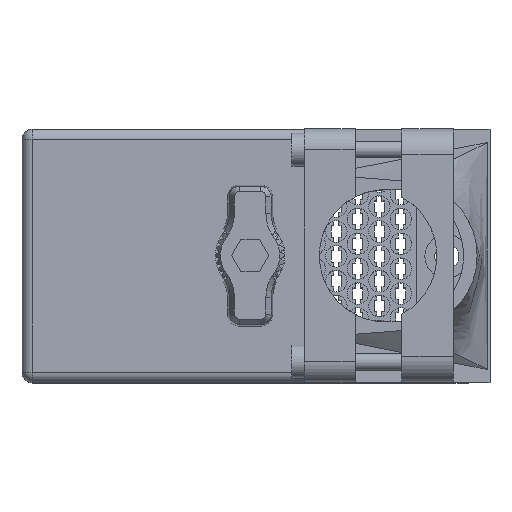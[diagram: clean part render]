
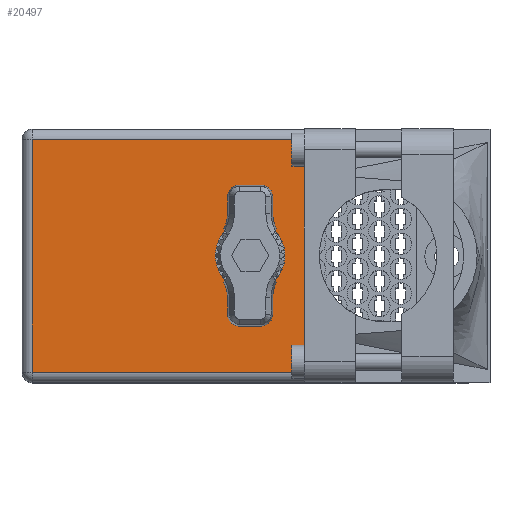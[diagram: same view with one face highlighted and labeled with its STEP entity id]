
A CAD part, top view. The second image highlights one B-rep face of the part: STEP entity #20497.
In plain terms, the highlighted face is planar.
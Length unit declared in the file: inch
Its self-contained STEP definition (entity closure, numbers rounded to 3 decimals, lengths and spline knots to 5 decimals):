
#471 = DIRECTION ( 'NONE',  ( 0., 1., 0. ) ) ;
#7063 = EDGE_CURVE ( 'NONE', #86197, #52435, #55895, .T. ) ;
#8745 = CIRCLE ( 'NONE', #77725, 0.1015 ) ;
#8870 = EDGE_CURVE ( 'NONE', #62942, #71681, #64493, .T. ) ;
#11421 = ORIENTED_EDGE ( 'NONE', *, *, #68523, .T. ) ;
#13861 = CARTESIAN_POINT ( 'NONE',  ( 1.705, 2.03, -1.468 ) ) ;
#15025 = CARTESIAN_POINT ( 'NONE',  ( 1.3775, 2.03, -0.8665 ) ) ;
#18262 = CARTESIAN_POINT ( 'NONE',  ( 0., 2.03, -1.53 ) ) ;
#19303 = DIRECTION ( 'NONE',  ( 0., 0., 1. ) ) ;
#19883 = CARTESIAN_POINT ( 'NONE',  ( 1.705, 2.03, -0.062 ) ) ;
#20497 = ADVANCED_FACE ( 'NONE', ( #49692, #53473 ), #90195, .T. ) ;
#23234 = LINE ( 'NONE', #57638, #63073 ) ;
#24453 = DIRECTION ( 'NONE',  ( 0., 0., 1. ) ) ;
#25493 = DIRECTION ( 'NONE',  ( 0., 1., 0. ) ) ;
#27387 = ORIENTED_EDGE ( 'NONE', *, *, #7063, .F. ) ;
#31021 = ORIENTED_EDGE ( 'NONE', *, *, #8870, .T. ) ;
#31385 = CARTESIAN_POINT ( 'NONE',  ( 1.3775, 2.03, -0.765 ) ) ;
#32904 = DIRECTION ( 'NONE',  ( 0., 0., 1. ) ) ;
#38269 = VERTEX_POINT ( 'NONE', #78449 ) ;
#42249 = LINE ( 'NONE', #99610, #59713 ) ;
#43285 = EDGE_CURVE ( 'NONE', #52435, #86197, #8745, .T. ) ;
#43323 = EDGE_LOOP ( 'NONE', ( #64674, #31021, #89694, #11421 ) ) ;
#43476 = AXIS2_PLACEMENT_3D ( 'NONE', #18262, #58951, #19303 ) ;
#45136 = CARTESIAN_POINT ( 'NONE',  ( 1.705, 2.03, -0.062 ) ) ;
#46689 = VECTOR ( 'NONE', #59989, 39.37008 ) ;
#49692 = FACE_OUTER_BOUND ( 'NONE', #43323, .T. ) ;
#52233 = DIRECTION ( 'NONE',  ( 1., 0., 0. ) ) ;
#52435 = VERTEX_POINT ( 'NONE', #101839 ) ;
#53005 = CARTESIAN_POINT ( 'NONE',  ( 0., 2.03, -1.468 ) ) ;
#53473 = FACE_BOUND ( 'NONE', #99322, .T. ) ;
#55895 = CIRCLE ( 'NONE', #74919, 0.1015 ) ;
#56486 = DIRECTION ( 'NONE',  ( 0., 0., 1. ) ) ;
#57638 = CARTESIAN_POINT ( 'NONE',  ( 0.062, 2.03, -1.53 ) ) ;
#58951 = DIRECTION ( 'NONE',  ( 0., 1., 0. ) ) ;
#59713 = VECTOR ( 'NONE', #61461, 39.37008 ) ;
#59989 = DIRECTION ( 'NONE',  ( -1., 0., 0. ) ) ;
#61098 = EDGE_CURVE ( 'NONE', #38269, #62942, #23234, .T. ) ;
#61461 = DIRECTION ( 'NONE',  ( 0., 0., 1. ) ) ;
#62942 = VERTEX_POINT ( 'NONE', #75344 ) ;
#63073 = VECTOR ( 'NONE', #32904, 39.37008 ) ;
#64493 = LINE ( 'NONE', #19883, #87925 ) ;
#64674 = ORIENTED_EDGE ( 'NONE', *, *, #61098, .T. ) ;
#64872 = VERTEX_POINT ( 'NONE', #13861 ) ;
#67815 = LINE ( 'NONE', #53005, #46689 ) ;
#68523 = EDGE_CURVE ( 'NONE', #64872, #38269, #67815, .T. ) ;
#71681 = VERTEX_POINT ( 'NONE', #45136 ) ;
#73126 = CARTESIAN_POINT ( 'NONE',  ( 1.3775, 2.03, -0.765 ) ) ;
#74919 = AXIS2_PLACEMENT_3D ( 'NONE', #73126, #25493, #56486 ) ;
#75344 = CARTESIAN_POINT ( 'NONE',  ( 0.062, 2.03, -0.062 ) ) ;
#77725 = AXIS2_PLACEMENT_3D ( 'NONE', #31385, #471, #24453 ) ;
#77867 = ORIENTED_EDGE ( 'NONE', *, *, #43285, .F. ) ;
#78449 = CARTESIAN_POINT ( 'NONE',  ( 0.062, 2.03, -1.468 ) ) ;
#86197 = VERTEX_POINT ( 'NONE', #15025 ) ;
#87925 = VECTOR ( 'NONE', #52233, 39.37008 ) ;
#89694 = ORIENTED_EDGE ( 'NONE', *, *, #102839, .F. ) ;
#90195 = PLANE ( 'NONE',  #43476 ) ;
#99322 = EDGE_LOOP ( 'NONE', ( #77867, #27387 ) ) ;
#99610 = CARTESIAN_POINT ( 'NONE',  ( 1.705, 2.03, -1.53 ) ) ;
#101839 = CARTESIAN_POINT ( 'NONE',  ( 1.3775, 2.03, -0.6635 ) ) ;
#102839 = EDGE_CURVE ( 'NONE', #64872, #71681, #42249, .T. ) ;
